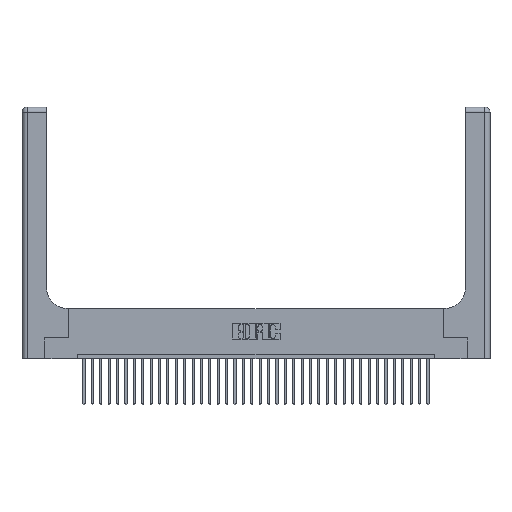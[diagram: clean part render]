
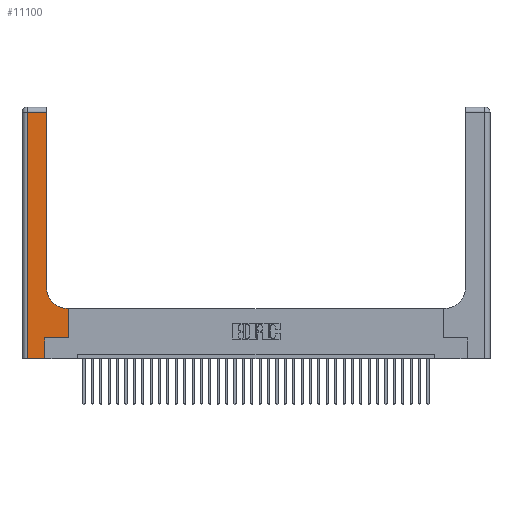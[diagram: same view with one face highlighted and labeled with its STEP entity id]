
A CAD part, top view. The second image highlights one B-rep face of the part: STEP entity #11100.
In plain terms, the highlighted planar face has unit normal (0, 0, 1).
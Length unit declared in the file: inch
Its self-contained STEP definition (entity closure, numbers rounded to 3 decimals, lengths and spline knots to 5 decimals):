
#841 = EDGE_LOOP ( 'NONE', ( #10919, #21212, #24780, #22975, #3704, #10135, #1889, #6807, #5921 ) ) ;
#1162 = EDGE_CURVE ( 'NONE', #11536, #6718, #1459, .T. ) ;
#1340 = CARTESIAN_POINT ( 'NONE',  ( 0.5415, 0.85, 0.37 ) ) ;
#1459 = LINE ( 'NONE', #15000, #32144 ) ;
#1630 = LINE ( 'NONE', #13009, #31853 ) ;
#1889 = ORIENTED_EDGE ( 'NONE', *, *, #33676, .T. ) ;
#2303 = DIRECTION ( 'NONE',  ( 0., -1., 0. ) ) ;
#2468 = VERTEX_POINT ( 'NONE', #27383 ) ;
#3704 = ORIENTED_EDGE ( 'NONE', *, *, #1162, .T. ) ;
#4329 = CARTESIAN_POINT ( 'NONE',  ( 0.269, 0., 0.37 ) ) ;
#4745 = DIRECTION ( 'NONE',  ( 1., 0., 0. ) ) ;
#4934 = DIRECTION ( 'NONE',  ( 0., 1., 0. ) ) ;
#5921 = ORIENTED_EDGE ( 'NONE', *, *, #20306, .T. ) ;
#6150 = LINE ( 'NONE', #16427, #15955 ) ;
#6591 = CARTESIAN_POINT ( 'NONE',  ( 0.269, 0.25, 0.37 ) ) ;
#6718 = VERTEX_POINT ( 'NONE', #6930 ) ;
#6801 = EDGE_CURVE ( 'NONE', #2468, #33043, #1630, .T. ) ;
#6807 = ORIENTED_EDGE ( 'NONE', *, *, #15831, .T. ) ;
#6871 = LINE ( 'NONE', #26301, #34406 ) ;
#6930 = CARTESIAN_POINT ( 'NONE',  ( 0.269, 0.25, 0.37 ) ) ;
#8186 = CARTESIAN_POINT ( 'NONE',  ( 0., 3., 0.37 ) ) ;
#8327 = CARTESIAN_POINT ( 'NONE',  ( 0.06, 0., 0.37 ) ) ;
#8419 = DIRECTION ( 'NONE',  ( -1., 0., 0. ) ) ;
#9505 = DIRECTION ( 'NONE',  ( 0., 1., 0. ) ) ;
#10089 = EDGE_CURVE ( 'NONE', #15670, #11536, #25338, .T. ) ;
#10135 = ORIENTED_EDGE ( 'NONE', *, *, #16942, .T. ) ;
#10165 = CARTESIAN_POINT ( 'NONE',  ( 0.5585, 0.25, 0.37 ) ) ;
#10919 = ORIENTED_EDGE ( 'NONE', *, *, #6801, .T. ) ;
#10962 = CARTESIAN_POINT ( 'NONE',  ( 0.5415, 0.6, 0.37 ) ) ;
#11100 = ADVANCED_FACE ( 'NONE', ( #32397 ), #13788, .F. ) ;
#11536 = VERTEX_POINT ( 'NONE', #4329 ) ;
#12082 = LINE ( 'NONE', #6591, #21408 ) ;
#12403 = DIRECTION ( 'NONE',  ( 1., 0., 0. ) ) ;
#12562 = CARTESIAN_POINT ( 'NONE',  ( 0.2915, 2.94, 0.37 ) ) ;
#13009 = CARTESIAN_POINT ( 'NONE',  ( 0.2915, 3., 0.37 ) ) ;
#13600 = LINE ( 'NONE', #15927, #27832 ) ;
#13788 = PLANE ( 'NONE',  #36621 ) ;
#13840 = VECTOR ( 'NONE', #4745, 39.37008 ) ;
#14537 = DIRECTION ( 'NONE',  ( 1., 0., 0. ) ) ;
#15000 = CARTESIAN_POINT ( 'NONE',  ( 0.269, 0., 0.37 ) ) ;
#15270 = DIRECTION ( 'NONE',  ( -1., 0., 0. ) ) ;
#15650 = DIRECTION ( 'NONE',  ( 0., 1., 0. ) ) ;
#15670 = VERTEX_POINT ( 'NONE', #8327 ) ;
#15831 = EDGE_CURVE ( 'NONE', #34264, #21360, #6871, .T. ) ;
#15927 = CARTESIAN_POINT ( 'NONE',  ( 0., 2.94, 0.37 ) ) ;
#15955 = VECTOR ( 'NONE', #2303, 39.37008 ) ;
#16354 = AXIS2_PLACEMENT_3D ( 'NONE', #1340, #23523, #12403 ) ;
#16427 = CARTESIAN_POINT ( 'NONE',  ( 0.06, 3., 0.37 ) ) ;
#16942 = EDGE_CURVE ( 'NONE', #6718, #34683, #12082, .T. ) ;
#19654 = VECTOR ( 'NONE', #15650, 39.37008 ) ;
#19745 = CARTESIAN_POINT ( 'NONE',  ( 0.06, 2.94, 0.37 ) ) ;
#20306 = EDGE_CURVE ( 'NONE', #21360, #2468, #21130, .T. ) ;
#21130 = CIRCLE ( 'NONE', #16354, 0.25 ) ;
#21212 = ORIENTED_EDGE ( 'NONE', *, *, #31488, .T. ) ;
#21360 = VERTEX_POINT ( 'NONE', #10962 ) ;
#21408 = VECTOR ( 'NONE', #14537, 39.37008 ) ;
#22679 = EDGE_CURVE ( 'NONE', #25289, #15670, #6150, .T. ) ;
#22975 = ORIENTED_EDGE ( 'NONE', *, *, #10089, .T. ) ;
#23523 = DIRECTION ( 'NONE',  ( 0., 0., -1. ) ) ;
#24780 = ORIENTED_EDGE ( 'NONE', *, *, #22679, .T. ) ;
#24983 = LINE ( 'NONE', #10165, #19654 ) ;
#25091 = CARTESIAN_POINT ( 'NONE',  ( 0., 0., 0.37 ) ) ;
#25289 = VERTEX_POINT ( 'NONE', #19745 ) ;
#25338 = LINE ( 'NONE', #25091, #13840 ) ;
#26301 = CARTESIAN_POINT ( 'NONE',  ( 0.2915, 0.6, 0.37 ) ) ;
#26353 = CARTESIAN_POINT ( 'NONE',  ( 0.5585, 0.25, 0.37 ) ) ;
#27028 = CARTESIAN_POINT ( 'NONE',  ( 0.5585, 0.6, 0.37 ) ) ;
#27383 = CARTESIAN_POINT ( 'NONE',  ( 0.2915, 0.85, 0.37 ) ) ;
#27832 = VECTOR ( 'NONE', #36034, 39.37008 ) ;
#28193 = DIRECTION ( 'NONE',  ( 0., 0., -1. ) ) ;
#31488 = EDGE_CURVE ( 'NONE', #33043, #25289, #13600, .T. ) ;
#31853 = VECTOR ( 'NONE', #4934, 39.37008 ) ;
#32144 = VECTOR ( 'NONE', #9505, 39.37008 ) ;
#32397 = FACE_OUTER_BOUND ( 'NONE', #841, .T. ) ;
#33043 = VERTEX_POINT ( 'NONE', #12562 ) ;
#33676 = EDGE_CURVE ( 'NONE', #34683, #34264, #24983, .T. ) ;
#34264 = VERTEX_POINT ( 'NONE', #27028 ) ;
#34406 = VECTOR ( 'NONE', #15270, 39.37008 ) ;
#34683 = VERTEX_POINT ( 'NONE', #26353 ) ;
#36034 = DIRECTION ( 'NONE',  ( -1., 0., 0. ) ) ;
#36621 = AXIS2_PLACEMENT_3D ( 'NONE', #8186, #28193, #8419 ) ;
